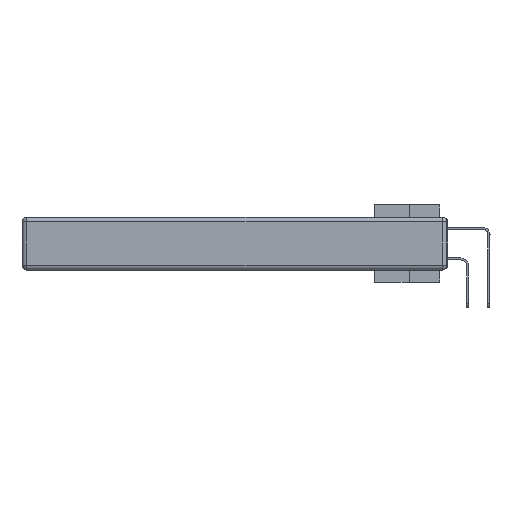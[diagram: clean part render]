
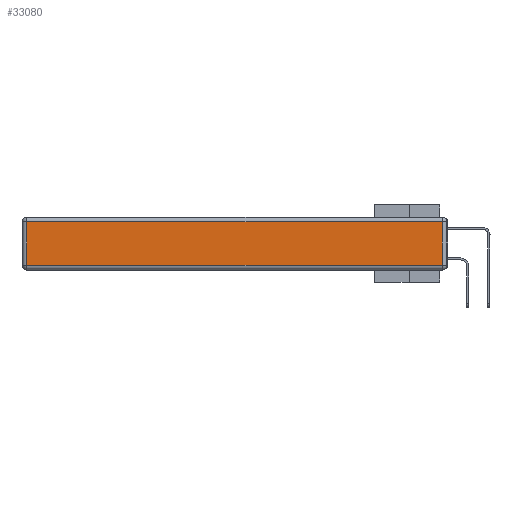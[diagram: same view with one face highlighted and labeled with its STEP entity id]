
A CAD part, left-side view. The second image highlights one B-rep face of the part: STEP entity #33080.
In plain terms, the highlighted planar face has unit normal (-1, 0, 0).
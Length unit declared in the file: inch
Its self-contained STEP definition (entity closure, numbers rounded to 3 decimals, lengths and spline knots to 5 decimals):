
#1088 = LINE ( 'NONE', #18340, #22473 ) ;
#1399 = DIRECTION ( 'NONE',  ( 0., 1., 0. ) ) ;
#1770 = VECTOR ( 'NONE', #1399, 39.37008 ) ;
#3474 = VERTEX_POINT ( 'NONE', #22681 ) ;
#4174 = LINE ( 'NONE', #7151, #14237 ) ;
#4706 = DIRECTION ( 'NONE',  ( 0., 0., -1. ) ) ;
#6220 = FACE_OUTER_BOUND ( 'NONE', #24237, .T. ) ;
#7151 = CARTESIAN_POINT ( 'NONE',  ( 0., 2.72, -0.343 ) ) ;
#7467 = DIRECTION ( 'NONE',  ( 0., 0., 1. ) ) ;
#7524 = VERTEX_POINT ( 'NONE', #28846 ) ;
#9613 = AXIS2_PLACEMENT_3D ( 'NONE', #22902, #14886, #12057 ) ;
#10685 = LINE ( 'NONE', #16503, #29470 ) ;
#11810 = PLANE ( 'NONE',  #9613 ) ;
#12057 = DIRECTION ( 'NONE',  ( 0., 0., 1. ) ) ;
#12908 = EDGE_CURVE ( 'NONE', #27019, #19311, #32354, .T. ) ;
#13139 = CARTESIAN_POINT ( 'NONE',  ( 0., 0.03, -0.03 ) ) ;
#14237 = VECTOR ( 'NONE', #4706, 39.37008 ) ;
#14886 = DIRECTION ( 'NONE',  ( -1., 0., 0. ) ) ;
#15115 = ORIENTED_EDGE ( 'NONE', *, *, #22875, .T. ) ;
#16503 = CARTESIAN_POINT ( 'NONE',  ( 0., 0., -0.313 ) ) ;
#18340 = CARTESIAN_POINT ( 'NONE',  ( 0., 0.03, -0.343 ) ) ;
#19095 = EDGE_CURVE ( 'NONE', #7524, #27019, #1088, .T. ) ;
#19311 = VERTEX_POINT ( 'NONE', #21602 ) ;
#19377 = ORIENTED_EDGE ( 'NONE', *, *, #19095, .T. ) ;
#19647 = DIRECTION ( 'NONE',  ( 0., -1., 0. ) ) ;
#21602 = CARTESIAN_POINT ( 'NONE',  ( 0., 2.72, -0.03 ) ) ;
#22473 = VECTOR ( 'NONE', #7467, 39.37008 ) ;
#22681 = CARTESIAN_POINT ( 'NONE',  ( 0., 2.72, -0.313 ) ) ;
#22875 = EDGE_CURVE ( 'NONE', #19311, #3474, #4174, .T. ) ;
#22902 = CARTESIAN_POINT ( 'NONE',  ( 0., 0., -0.343 ) ) ;
#24237 = EDGE_LOOP ( 'NONE', ( #24324, #19377, #29692, #15115 ) ) ;
#24324 = ORIENTED_EDGE ( 'NONE', *, *, #29818, .T. ) ;
#27019 = VERTEX_POINT ( 'NONE', #13139 ) ;
#28846 = CARTESIAN_POINT ( 'NONE',  ( 0., 0.03, -0.313 ) ) ;
#29470 = VECTOR ( 'NONE', #19647, 39.37008 ) ;
#29692 = ORIENTED_EDGE ( 'NONE', *, *, #12908, .T. ) ;
#29726 = CARTESIAN_POINT ( 'NONE',  ( 0., 2.75, -0.03 ) ) ;
#29818 = EDGE_CURVE ( 'NONE', #3474, #7524, #10685, .T. ) ;
#32354 = LINE ( 'NONE', #29726, #1770 ) ;
#33080 = ADVANCED_FACE ( 'NONE', ( #6220 ), #11810, .T. ) ;
